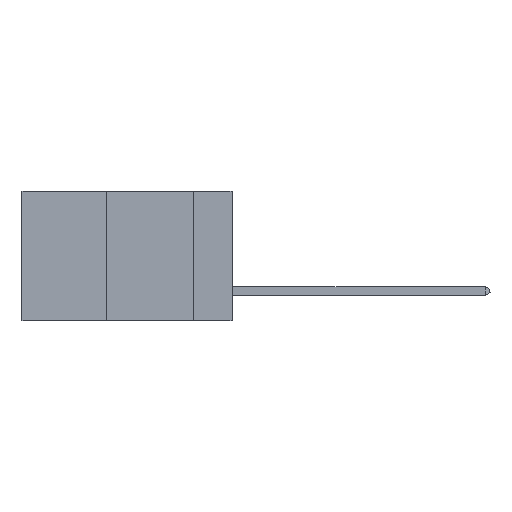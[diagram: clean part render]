
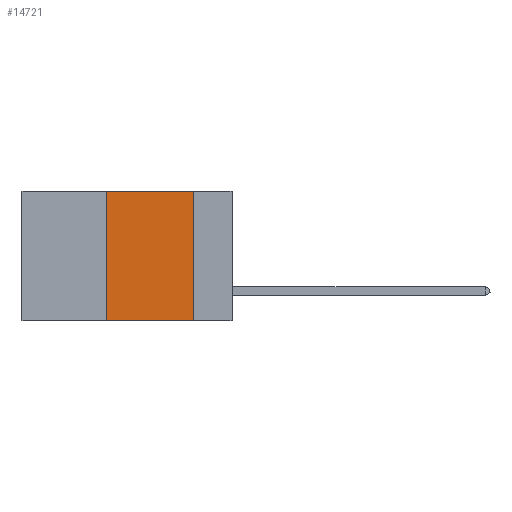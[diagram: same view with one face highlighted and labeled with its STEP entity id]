
A CAD part, left-side view. The second image highlights one B-rep face of the part: STEP entity #14721.
In plain terms, the highlighted planar face has unit normal (-1, 0, 0).
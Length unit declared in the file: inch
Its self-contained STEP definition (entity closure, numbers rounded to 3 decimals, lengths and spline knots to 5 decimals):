
#2152 = EDGE_CURVE ( 'NONE', #9996, #21060, #15194, .T. ) ;
#4135 = EDGE_CURVE ( 'NONE', #8291, #17699, #12577, .T. ) ;
#4473 = VECTOR ( 'NONE', #10605, 39.37008 ) ;
#4516 = CARTESIAN_POINT ( 'NONE',  ( 0., 0.36, -0.37 ) ) ;
#4766 = CARTESIAN_POINT ( 'NONE',  ( 0., 0.6, -0.37 ) ) ;
#4895 = VECTOR ( 'NONE', #15416, 39.37008 ) ;
#6450 = DIRECTION ( 'NONE',  ( 1., 0., 0. ) ) ;
#6580 = ORIENTED_EDGE ( 'NONE', *, *, #6826, .F. ) ;
#6826 = EDGE_CURVE ( 'NONE', #8291, #9996, #16092, .T. ) ;
#6866 = CARTESIAN_POINT ( 'NONE',  ( 0., 0.36, 0. ) ) ;
#7282 = ORIENTED_EDGE ( 'NONE', *, *, #4135, .T. ) ;
#7805 = VECTOR ( 'NONE', #8614, 39.37008 ) ;
#8291 = VERTEX_POINT ( 'NONE', #4516 ) ;
#8547 = VECTOR ( 'NONE', #22775, 39.37008 ) ;
#8614 = DIRECTION ( 'NONE',  ( 0., 0., 1. ) ) ;
#9996 = VERTEX_POINT ( 'NONE', #11009 ) ;
#10605 = DIRECTION ( 'NONE',  ( 0., 0., -1. ) ) ;
#11009 = CARTESIAN_POINT ( 'NONE',  ( 0., 0.36, 0. ) ) ;
#11105 = ORIENTED_EDGE ( 'NONE', *, *, #13777, .F. ) ;
#12062 = CARTESIAN_POINT ( 'NONE',  ( 0., 0.11, 0. ) ) ;
#12577 = LINE ( 'NONE', #4766, #4895 ) ;
#13130 = CARTESIAN_POINT ( 'NONE',  ( 0., 0.6, 0. ) ) ;
#13777 = EDGE_CURVE ( 'NONE', #21060, #17699, #18278, .T. ) ;
#14026 = CARTESIAN_POINT ( 'NONE',  ( 0., 0.11, 0. ) ) ;
#14721 = ADVANCED_FACE ( 'NONE', ( #16293 ), #18382, .F. ) ;
#15194 = LINE ( 'NONE', #19236, #8547 ) ;
#15416 = DIRECTION ( 'NONE',  ( 0., -1., 0. ) ) ;
#15641 = CARTESIAN_POINT ( 'NONE',  ( 0., 0.11, -0.37 ) ) ;
#16092 = LINE ( 'NONE', #6866, #7805 ) ;
#16293 = FACE_OUTER_BOUND ( 'NONE', #20674, .T. ) ;
#17699 = VERTEX_POINT ( 'NONE', #15641 ) ;
#18278 = LINE ( 'NONE', #14026, #4473 ) ;
#18382 = PLANE ( 'NONE',  #22159 ) ;
#19236 = CARTESIAN_POINT ( 'NONE',  ( 0., 0.6, 0. ) ) ;
#20674 = EDGE_LOOP ( 'NONE', ( #11105, #20968, #6580, #7282 ) ) ;
#20968 = ORIENTED_EDGE ( 'NONE', *, *, #2152, .F. ) ;
#21060 = VERTEX_POINT ( 'NONE', #12062 ) ;
#22159 = AXIS2_PLACEMENT_3D ( 'NONE', #13130, #6450, #22300 ) ;
#22300 = DIRECTION ( 'NONE',  ( 0., 0., -1. ) ) ;
#22775 = DIRECTION ( 'NONE',  ( 0., -1., 0. ) ) ;
